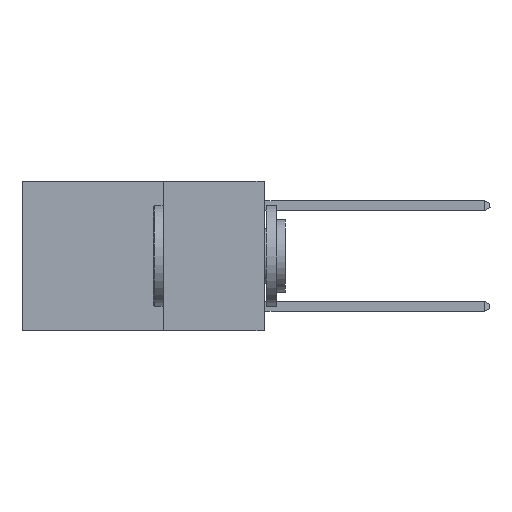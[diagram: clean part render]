
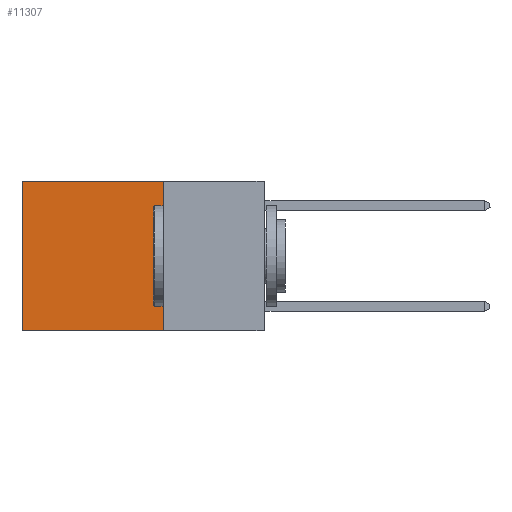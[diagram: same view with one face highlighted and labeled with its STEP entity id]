
A CAD part, left-side view. The second image highlights one B-rep face of the part: STEP entity #11307.
In plain terms, the highlighted planar face has unit normal (-1, 0, 0).
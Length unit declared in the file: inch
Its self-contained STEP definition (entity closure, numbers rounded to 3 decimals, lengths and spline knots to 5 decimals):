
#150 = EDGE_CURVE ( 'NONE', #12145, #11991, #15505, .T. ) ;
#1098 = CARTESIAN_POINT ( 'NONE',  ( 0.2625, 0.25, 0. ) ) ;
#1442 = CARTESIAN_POINT ( 'NONE',  ( 0.2625, 0.25, 0. ) ) ;
#1766 = LINE ( 'NONE', #12825, #11089 ) ;
#3116 = EDGE_CURVE ( 'NONE', #7376, #11991, #10640, .T. ) ;
#3578 = CARTESIAN_POINT ( 'NONE',  ( 0.2625, 0.6, 0. ) ) ;
#3941 = DIRECTION ( 'NONE',  ( 0., 0., -1. ) ) ;
#5625 = CARTESIAN_POINT ( 'NONE',  ( 0.2625, 0.25, 0. ) ) ;
#6366 = CARTESIAN_POINT ( 'NONE',  ( 0.2625, 0.25, -0.37 ) ) ;
#6480 = DIRECTION ( 'NONE',  ( 0., 1., 0. ) ) ;
#6840 = DIRECTION ( 'NONE',  ( 0., 0., -1. ) ) ;
#7357 = CARTESIAN_POINT ( 'NONE',  ( 0.2625, 0.6, -0.37 ) ) ;
#7376 = VERTEX_POINT ( 'NONE', #3578 ) ;
#7458 = VECTOR ( 'NONE', #13944, 39.37008 ) ;
#7925 = ORIENTED_EDGE ( 'NONE', *, *, #11900, .T. ) ;
#8117 = LINE ( 'NONE', #1098, #14057 ) ;
#8504 = FACE_OUTER_BOUND ( 'NONE', #13957, .T. ) ;
#9064 = ORIENTED_EDGE ( 'NONE', *, *, #3116, .T. ) ;
#9702 = ORIENTED_EDGE ( 'NONE', *, *, #150, .F. ) ;
#9976 = PLANE ( 'NONE',  #15587 ) ;
#10640 = LINE ( 'NONE', #15019, #7458 ) ;
#11089 = VECTOR ( 'NONE', #6840, 39.37008 ) ;
#11201 = DIRECTION ( 'NONE',  ( 1., 0., 0. ) ) ;
#11307 = ADVANCED_FACE ( 'NONE', ( #8504 ), #9976, .F. ) ;
#11591 = EDGE_CURVE ( 'NONE', #12301, #12145, #1766, .T. ) ;
#11644 = ORIENTED_EDGE ( 'NONE', *, *, #11591, .F. ) ;
#11900 = EDGE_CURVE ( 'NONE', #12301, #7376, #8117, .T. ) ;
#11991 = VERTEX_POINT ( 'NONE', #7357 ) ;
#12036 = DIRECTION ( 'NONE',  ( 0., 1., 0. ) ) ;
#12145 = VERTEX_POINT ( 'NONE', #6366 ) ;
#12301 = VERTEX_POINT ( 'NONE', #5625 ) ;
#12440 = VECTOR ( 'NONE', #6480, 39.37008 ) ;
#12825 = CARTESIAN_POINT ( 'NONE',  ( 0.2625, 0.25, 0. ) ) ;
#12928 = CARTESIAN_POINT ( 'NONE',  ( 0.2625, 0.25, -0.37 ) ) ;
#13944 = DIRECTION ( 'NONE',  ( 0., 0., -1. ) ) ;
#13957 = EDGE_LOOP ( 'NONE', ( #9064, #9702, #11644, #7925 ) ) ;
#14057 = VECTOR ( 'NONE', #12036, 39.37008 ) ;
#15019 = CARTESIAN_POINT ( 'NONE',  ( 0.2625, 0.6, 0. ) ) ;
#15505 = LINE ( 'NONE', #12928, #12440 ) ;
#15587 = AXIS2_PLACEMENT_3D ( 'NONE', #1442, #11201, #3941 ) ;
